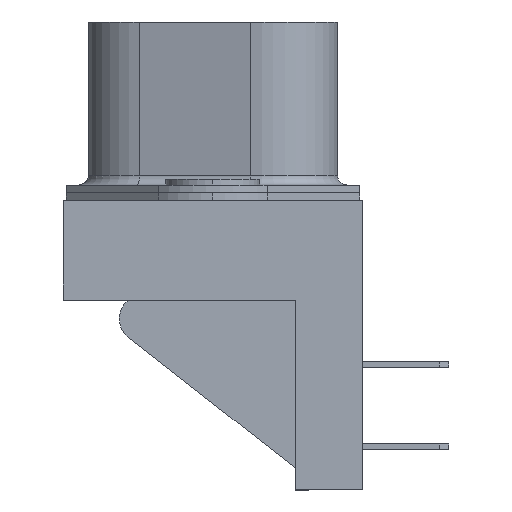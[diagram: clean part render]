
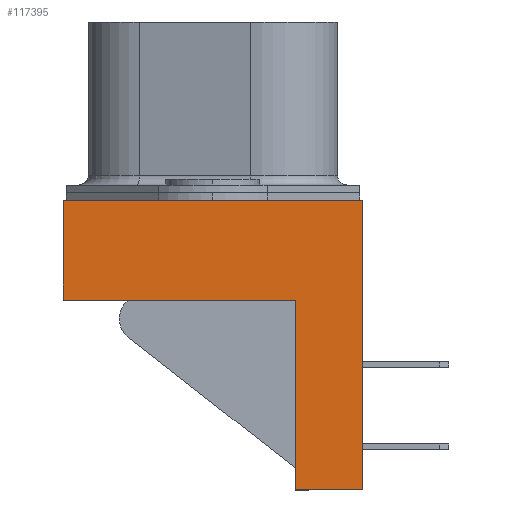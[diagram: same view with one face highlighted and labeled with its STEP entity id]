
A CAD part, left-side view. The second image highlights one B-rep face of the part: STEP entity #117395.
In plain terms, the highlighted planar face has unit normal (-1, 0, 0).
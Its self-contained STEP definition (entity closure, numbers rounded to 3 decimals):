
#947 = DIRECTION ( 'NONE',  ( 0., 1., 0. ) ) ;
#2810 = LINE ( 'NONE', #19798, #162527 ) ;
#3087 = LINE ( 'NONE', #110782, #103178 ) ;
#6078 = CARTESIAN_POINT ( 'NONE',  ( -4.125, -7.8, -15.1 ) ) ;
#10878 = VERTEX_POINT ( 'NONE', #6078 ) ;
#16602 = VECTOR ( 'NONE', #114238, 1000. ) ;
#18744 = DIRECTION ( 'NONE',  ( 0., -1., 0. ) ) ;
#19798 = CARTESIAN_POINT ( 'NONE',  ( -4.125, 7.8, -15.1 ) ) ;
#31669 = CARTESIAN_POINT ( 'NONE',  ( -4.125, -7.8, -15.1 ) ) ;
#33084 = LINE ( 'NONE', #100365, #84489 ) ;
#35066 = EDGE_CURVE ( 'NONE', #149476, #10878, #33084, .T. ) ;
#36148 = AXIS2_PLACEMENT_3D ( 'NONE', #147997, #109426, #95969 ) ;
#37686 = PLANE ( 'NONE',  #36148 ) ;
#49657 = ORIENTED_EDGE ( 'NONE', *, *, #78988, .F. ) ;
#51935 = ORIENTED_EDGE ( 'NONE', *, *, #35066, .T. ) ;
#53154 = VECTOR ( 'NONE', #146257, 1000. ) ;
#54673 = FACE_OUTER_BOUND ( 'NONE', #95850, .T. ) ;
#57499 = EDGE_CURVE ( 'NONE', #105740, #127492, #78999, .T. ) ;
#60365 = LINE ( 'NONE', #31669, #16602 ) ;
#61209 = VERTEX_POINT ( 'NONE', #68622 ) ;
#68622 = CARTESIAN_POINT ( 'NONE',  ( -4.125, -4.3, -5.2 ) ) ;
#71591 = ORIENTED_EDGE ( 'NONE', *, *, #57499, .F. ) ;
#72765 = CARTESIAN_POINT ( 'NONE',  ( -4.125, -7.8, 0. ) ) ;
#75439 = EDGE_CURVE ( 'NONE', #10878, #127492, #60365, .T. ) ;
#78988 = EDGE_CURVE ( 'NONE', #149476, #61209, #3087, .T. ) ;
#78999 = LINE ( 'NONE', #120278, #53154 ) ;
#83812 = DIRECTION ( 'NONE',  ( 0., 0., 1. ) ) ;
#84489 = VECTOR ( 'NONE', #18744, 1000. ) ;
#86367 = CARTESIAN_POINT ( 'NONE',  ( -4.125, 7.8, 0. ) ) ;
#94254 = LINE ( 'NONE', #176753, #170679 ) ;
#95850 = EDGE_LOOP ( 'NONE', ( #95919, #49657, #51935, #130684, #71591, #120553 ) ) ;
#95919 = ORIENTED_EDGE ( 'NONE', *, *, #170102, .F. ) ;
#95969 = DIRECTION ( 'NONE',  ( 0., -1., 0. ) ) ;
#100365 = CARTESIAN_POINT ( 'NONE',  ( -4.125, 7.8, -15.1 ) ) ;
#103178 = VECTOR ( 'NONE', #83812, 1000. ) ;
#105740 = VERTEX_POINT ( 'NONE', #86367 ) ;
#108643 = CARTESIAN_POINT ( 'NONE',  ( -4.125, 7.8, -5.2 ) ) ;
#109426 = DIRECTION ( 'NONE',  ( -1., 0., 0. ) ) ;
#110782 = CARTESIAN_POINT ( 'NONE',  ( -4.125, -4.3, -15.1 ) ) ;
#114238 = DIRECTION ( 'NONE',  ( 0., 0., 1. ) ) ;
#117395 = ADVANCED_FACE ( 'NONE', ( #54673 ), #37686, .T. ) ;
#120278 = CARTESIAN_POINT ( 'NONE',  ( -4.125, 7.8, 0. ) ) ;
#120553 = ORIENTED_EDGE ( 'NONE', *, *, #151979, .F. ) ;
#127492 = VERTEX_POINT ( 'NONE', #72765 ) ;
#130684 = ORIENTED_EDGE ( 'NONE', *, *, #75439, .T. ) ;
#141780 = DIRECTION ( 'NONE',  ( 0., 0., 1. ) ) ;
#146257 = DIRECTION ( 'NONE',  ( 0., -1., 0. ) ) ;
#147997 = CARTESIAN_POINT ( 'NONE',  ( -4.125, 7.8, -15.1 ) ) ;
#149476 = VERTEX_POINT ( 'NONE', #162245 ) ;
#151979 = EDGE_CURVE ( 'NONE', #174351, #105740, #2810, .T. ) ;
#162245 = CARTESIAN_POINT ( 'NONE',  ( -4.125, -4.3, -15.1 ) ) ;
#162527 = VECTOR ( 'NONE', #141780, 1000. ) ;
#170102 = EDGE_CURVE ( 'NONE', #61209, #174351, #94254, .T. ) ;
#170679 = VECTOR ( 'NONE', #947, 1000. ) ;
#174351 = VERTEX_POINT ( 'NONE', #108643 ) ;
#176753 = CARTESIAN_POINT ( 'NONE',  ( -4.125, 7.8, -5.2 ) ) ;
